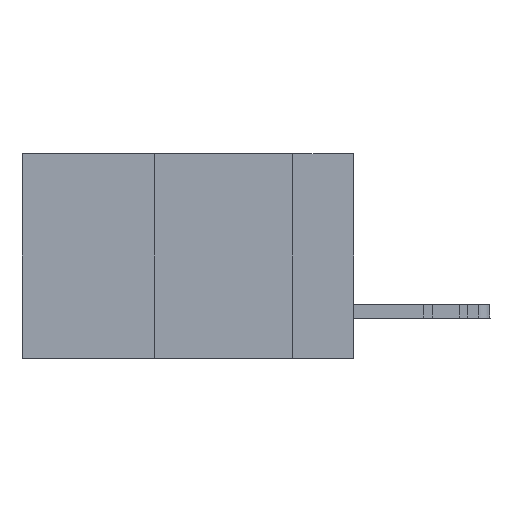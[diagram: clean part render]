
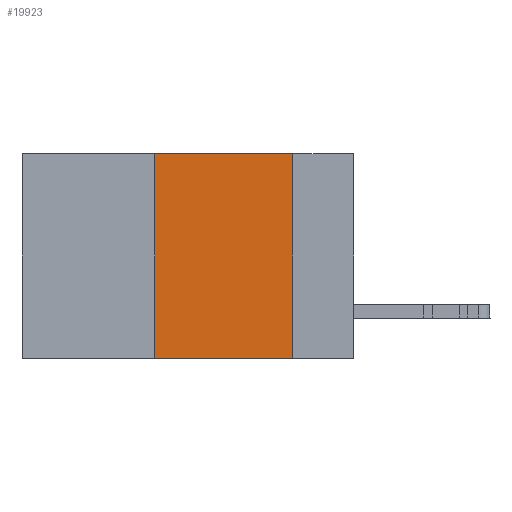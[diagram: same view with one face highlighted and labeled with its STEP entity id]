
A CAD part, left-side view. The second image highlights one B-rep face of the part: STEP entity #19923.
In plain terms, the highlighted planar face has unit normal (-1, 0, 0).
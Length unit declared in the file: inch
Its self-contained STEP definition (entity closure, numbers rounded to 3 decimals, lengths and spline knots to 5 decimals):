
#1981 = ORIENTED_EDGE ( 'NONE', *, *, #43662, .T. ) ;
#3562 = VERTEX_POINT ( 'NONE', #31532 ) ;
#4175 = CARTESIAN_POINT ( 'NONE',  ( 0., 0.6, 0. ) ) ;
#4504 = DIRECTION ( 'NONE',  ( 0., -1., 0. ) ) ;
#4772 = AXIS2_PLACEMENT_3D ( 'NONE', #37395, #15227, #10975 ) ;
#4830 = ORIENTED_EDGE ( 'NONE', *, *, #48231, .F. ) ;
#6478 = DIRECTION ( 'NONE',  ( 0., 0., 1. ) ) ;
#6781 = CARTESIAN_POINT ( 'NONE',  ( 0., 0.11, 0. ) ) ;
#8246 = EDGE_CURVE ( 'NONE', #10911, #26915, #42260, .T. ) ;
#10911 = VERTEX_POINT ( 'NONE', #6781 ) ;
#10975 = DIRECTION ( 'NONE',  ( 0., 0., -1. ) ) ;
#11197 = ORIENTED_EDGE ( 'NONE', *, *, #40783, .F. ) ;
#11523 = VECTOR ( 'NONE', #29089, 39.37008 ) ;
#15227 = DIRECTION ( 'NONE',  ( 1., 0., 0. ) ) ;
#16318 = VECTOR ( 'NONE', #46707, 39.37008 ) ;
#19923 = ADVANCED_FACE ( 'NONE', ( #35643 ), #25967, .F. ) ;
#20255 = CARTESIAN_POINT ( 'NONE',  ( 0., 0.6, -0.37 ) ) ;
#22801 = ORIENTED_EDGE ( 'NONE', *, *, #8246, .F. ) ;
#22914 = LINE ( 'NONE', #44133, #27002 ) ;
#25967 = PLANE ( 'NONE',  #4772 ) ;
#26915 = VERTEX_POINT ( 'NONE', #36391 ) ;
#27002 = VECTOR ( 'NONE', #6478, 39.37008 ) ;
#28908 = VERTEX_POINT ( 'NONE', #42101 ) ;
#29089 = DIRECTION ( 'NONE',  ( 0., 0., -1. ) ) ;
#31532 = CARTESIAN_POINT ( 'NONE',  ( 0., 0.36, -0.37 ) ) ;
#32681 = EDGE_LOOP ( 'NONE', ( #22801, #11197, #4830, #1981 ) ) ;
#32829 = LINE ( 'NONE', #20255, #16318 ) ;
#34689 = VECTOR ( 'NONE', #4504, 39.37008 ) ;
#35643 = FACE_OUTER_BOUND ( 'NONE', #32681, .T. ) ;
#35880 = LINE ( 'NONE', #4175, #34689 ) ;
#36391 = CARTESIAN_POINT ( 'NONE',  ( 0., 0.11, -0.37 ) ) ;
#37395 = CARTESIAN_POINT ( 'NONE',  ( 0., 0.6, 0. ) ) ;
#40783 = EDGE_CURVE ( 'NONE', #28908, #10911, #35880, .T. ) ;
#42101 = CARTESIAN_POINT ( 'NONE',  ( 0., 0.36, 0. ) ) ;
#42260 = LINE ( 'NONE', #48278, #11523 ) ;
#43662 = EDGE_CURVE ( 'NONE', #3562, #26915, #32829, .T. ) ;
#44133 = CARTESIAN_POINT ( 'NONE',  ( 0., 0.36, 0. ) ) ;
#46707 = DIRECTION ( 'NONE',  ( 0., -1., 0. ) ) ;
#48231 = EDGE_CURVE ( 'NONE', #3562, #28908, #22914, .T. ) ;
#48278 = CARTESIAN_POINT ( 'NONE',  ( 0., 0.11, 0. ) ) ;
